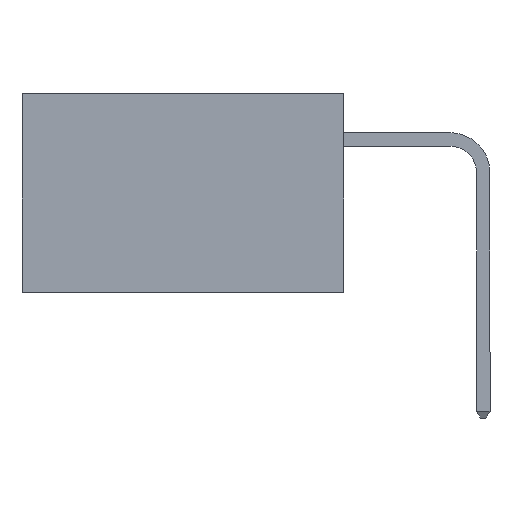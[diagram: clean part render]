
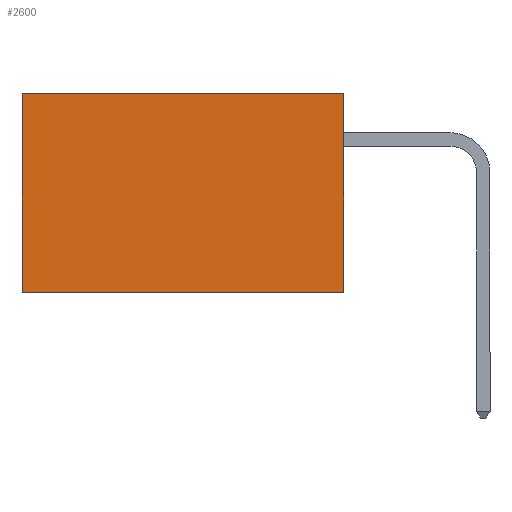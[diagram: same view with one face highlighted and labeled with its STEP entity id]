
A CAD part, left-side view. The second image highlights one B-rep face of the part: STEP entity #2600.
In plain terms, the highlighted planar face has unit normal (-1, 0, 0).
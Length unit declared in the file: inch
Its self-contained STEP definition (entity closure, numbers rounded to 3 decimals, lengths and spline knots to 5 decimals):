
#293 = LINE ( 'NONE', #5574, #552 ) ;
#552 = VECTOR ( 'NONE', #2348, 39.37008 ) ;
#561 = AXIS2_PLACEMENT_3D ( 'NONE', #6237, #4449, #2402 ) ;
#622 = LINE ( 'NONE', #7265, #5993 ) ;
#935 = VERTEX_POINT ( 'NONE', #3856 ) ;
#1074 = CARTESIAN_POINT ( 'NONE',  ( 0.2615, 0., -0.37 ) ) ;
#1373 = CARTESIAN_POINT ( 'NONE',  ( 0.2615, 0., -0.37 ) ) ;
#1545 = CARTESIAN_POINT ( 'NONE',  ( 0.2615, 0., 0. ) ) ;
#2348 = DIRECTION ( 'NONE',  ( 0., 1., 0. ) ) ;
#2402 = DIRECTION ( 'NONE',  ( 0., 0., -1. ) ) ;
#2600 = ADVANCED_FACE ( 'NONE', ( #2977 ), #7044, .F. ) ;
#2790 = VECTOR ( 'NONE', #6416, 39.37008 ) ;
#2977 = FACE_OUTER_BOUND ( 'NONE', #7173, .T. ) ;
#3753 = CARTESIAN_POINT ( 'NONE',  ( 0.2615, 0., -0.37 ) ) ;
#3774 = VERTEX_POINT ( 'NONE', #5819 ) ;
#3856 = CARTESIAN_POINT ( 'NONE',  ( 0.2615, 0.6, -0.37 ) ) ;
#3923 = VECTOR ( 'NONE', #6462, 39.37008 ) ;
#3995 = ORIENTED_EDGE ( 'NONE', *, *, #8444, .F. ) ;
#4449 = DIRECTION ( 'NONE',  ( 1., 0., 0. ) ) ;
#4608 = EDGE_CURVE ( 'NONE', #7430, #6804, #8545, .T. ) ;
#5574 = CARTESIAN_POINT ( 'NONE',  ( 0.2615, 0., 0. ) ) ;
#5622 = ORIENTED_EDGE ( 'NONE', *, *, #4608, .F. ) ;
#5817 = DIRECTION ( 'NONE',  ( 0., 0., -1. ) ) ;
#5819 = CARTESIAN_POINT ( 'NONE',  ( 0.2615, 0.6, 0. ) ) ;
#5993 = VECTOR ( 'NONE', #5817, 39.37008 ) ;
#6237 = CARTESIAN_POINT ( 'NONE',  ( 0.2615, 0., -0.37 ) ) ;
#6416 = DIRECTION ( 'NONE',  ( 0., 1., 0. ) ) ;
#6462 = DIRECTION ( 'NONE',  ( 0., 0., -1. ) ) ;
#6804 = VERTEX_POINT ( 'NONE', #1373 ) ;
#7044 = PLANE ( 'NONE',  #561 ) ;
#7173 = EDGE_LOOP ( 'NONE', ( #8434, #3995, #5622, #7375 ) ) ;
#7265 = CARTESIAN_POINT ( 'NONE',  ( 0.2615, 0.6, -0.37 ) ) ;
#7375 = ORIENTED_EDGE ( 'NONE', *, *, #8428, .T. ) ;
#7430 = VERTEX_POINT ( 'NONE', #1545 ) ;
#7687 = LINE ( 'NONE', #3753, #2790 ) ;
#8156 = EDGE_CURVE ( 'NONE', #3774, #935, #622, .T. ) ;
#8428 = EDGE_CURVE ( 'NONE', #7430, #3774, #293, .T. ) ;
#8434 = ORIENTED_EDGE ( 'NONE', *, *, #8156, .T. ) ;
#8444 = EDGE_CURVE ( 'NONE', #6804, #935, #7687, .T. ) ;
#8545 = LINE ( 'NONE', #1074, #3923 ) ;
